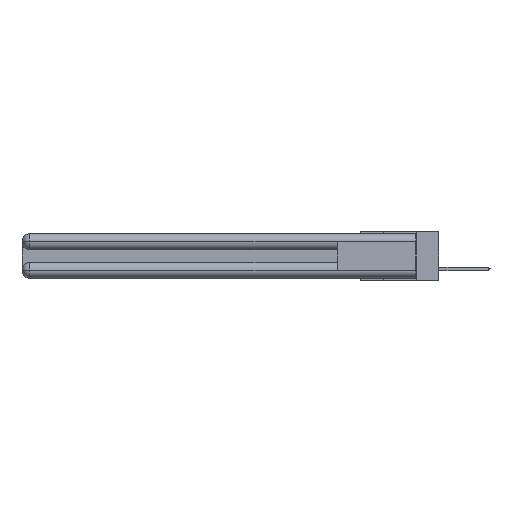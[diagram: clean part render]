
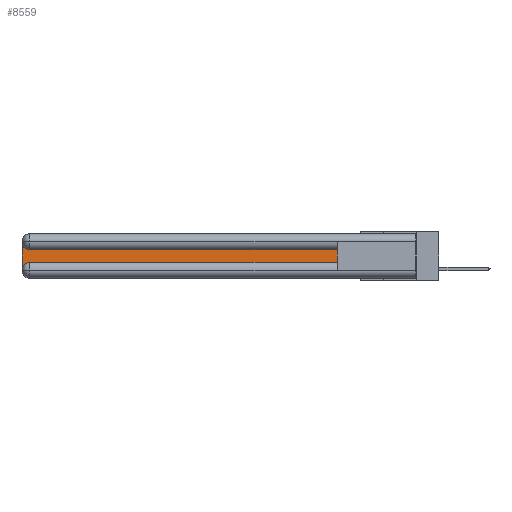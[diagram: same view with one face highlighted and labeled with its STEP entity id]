
A CAD part, left-side view. The second image highlights one B-rep face of the part: STEP entity #8559.
In plain terms, the highlighted planar face has unit normal (-1, 0, 0).
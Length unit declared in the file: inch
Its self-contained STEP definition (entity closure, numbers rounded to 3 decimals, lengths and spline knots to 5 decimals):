
#857 = DIRECTION ( 'NONE',  ( 0., 1., 0. ) ) ;
#1950 = EDGE_CURVE ( 'NONE', #27171, #4765, #4205, .T. ) ;
#3965 = VERTEX_POINT ( 'NONE', #7953 ) ;
#4006 = CARTESIAN_POINT ( 'NONE',  ( 0.075, 2.94, -0.1225 ) ) ;
#4038 = CARTESIAN_POINT ( 'NONE',  ( 0.075, 0.6, -0.1225 ) ) ;
#4043 = ORIENTED_EDGE ( 'NONE', *, *, #16561, .T. ) ;
#4205 = CIRCLE ( 'NONE', #23764, 0.06 ) ;
#4765 = VERTEX_POINT ( 'NONE', #13547 ) ;
#4805 = ORIENTED_EDGE ( 'NONE', *, *, #29061, .T. ) ;
#5622 = CARTESIAN_POINT ( 'NONE',  ( 0.075, 3., -0.2775 ) ) ;
#5799 = EDGE_CURVE ( 'NONE', #27589, #27171, #24409, .T. ) ;
#6593 = VERTEX_POINT ( 'NONE', #4006 ) ;
#6623 = VECTOR ( 'NONE', #11444, 39.37008 ) ;
#6762 = FACE_OUTER_BOUND ( 'NONE', #28448, .T. ) ;
#7567 = DIRECTION ( 'NONE',  ( 0., 0., -1. ) ) ;
#7831 = AXIS2_PLACEMENT_3D ( 'NONE', #11218, #16255, #26977 ) ;
#7953 = CARTESIAN_POINT ( 'NONE',  ( 0.075, 0.6, -0.2175 ) ) ;
#8559 = ADVANCED_FACE ( 'NONE', ( #6762 ), #8961, .F. ) ;
#8961 = PLANE ( 'NONE',  #7831 ) ;
#9334 = AXIS2_PLACEMENT_3D ( 'NONE', #18799, #28053, #7567 ) ;
#11218 = CARTESIAN_POINT ( 'NONE',  ( 0.075, 3., -0.1225 ) ) ;
#11444 = DIRECTION ( 'NONE',  ( 0., 0., 1. ) ) ;
#11718 = VERTEX_POINT ( 'NONE', #4038 ) ;
#12567 = VECTOR ( 'NONE', #15115, 39.37008 ) ;
#12630 = ORIENTED_EDGE ( 'NONE', *, *, #5799, .T. ) ;
#13535 = CARTESIAN_POINT ( 'NONE',  ( 0.075, 2.94, -0.2775 ) ) ;
#13547 = CARTESIAN_POINT ( 'NONE',  ( 0.075, 2.94, -0.2175 ) ) ;
#14066 = LINE ( 'NONE', #14247, #16212 ) ;
#14247 = CARTESIAN_POINT ( 'NONE',  ( 0.075, 0.6, -0.1225 ) ) ;
#15014 = CIRCLE ( 'NONE', #9334, 0.06 ) ;
#15115 = DIRECTION ( 'NONE',  ( 0., -1., 0. ) ) ;
#15413 = LINE ( 'NONE', #24854, #6623 ) ;
#15864 = DIRECTION ( 'NONE',  ( 0., 0., -1. ) ) ;
#16137 = ORIENTED_EDGE ( 'NONE', *, *, #26480, .T. ) ;
#16212 = VECTOR ( 'NONE', #857, 39.37008 ) ;
#16213 = DIRECTION ( 'NONE',  ( 1., 0., 0. ) ) ;
#16255 = DIRECTION ( 'NONE',  ( 1., 0., 0. ) ) ;
#16296 = VECTOR ( 'NONE', #15864, 39.37008 ) ;
#16561 = EDGE_CURVE ( 'NONE', #3965, #11718, #15413, .T. ) ;
#18181 = CARTESIAN_POINT ( 'NONE',  ( 0.075, 3., -0.0625 ) ) ;
#18280 = DIRECTION ( 'NONE',  ( 0., 0., -1. ) ) ;
#18552 = ORIENTED_EDGE ( 'NONE', *, *, #1950, .T. ) ;
#18587 = LINE ( 'NONE', #24377, #12567 ) ;
#18799 = CARTESIAN_POINT ( 'NONE',  ( 0.075, 2.94, -0.0625 ) ) ;
#22326 = ORIENTED_EDGE ( 'NONE', *, *, #27195, .T. ) ;
#22876 = CARTESIAN_POINT ( 'NONE',  ( 0.075, 3., -0.2175 ) ) ;
#23764 = AXIS2_PLACEMENT_3D ( 'NONE', #13535, #16213, #18280 ) ;
#24377 = CARTESIAN_POINT ( 'NONE',  ( 0.075, 0.6, -0.2175 ) ) ;
#24409 = LINE ( 'NONE', #22876, #16296 ) ;
#24854 = CARTESIAN_POINT ( 'NONE',  ( 0.075, 0.6, -0.2175 ) ) ;
#26480 = EDGE_CURVE ( 'NONE', #4765, #3965, #18587, .T. ) ;
#26977 = DIRECTION ( 'NONE',  ( 0., 0., -1. ) ) ;
#27171 = VERTEX_POINT ( 'NONE', #5622 ) ;
#27195 = EDGE_CURVE ( 'NONE', #6593, #27589, #15014, .T. ) ;
#27589 = VERTEX_POINT ( 'NONE', #18181 ) ;
#28053 = DIRECTION ( 'NONE',  ( 1., 0., 0. ) ) ;
#28448 = EDGE_LOOP ( 'NONE', ( #4805, #22326, #12630, #18552, #16137, #4043 ) ) ;
#29061 = EDGE_CURVE ( 'NONE', #11718, #6593, #14066, .T. ) ;
